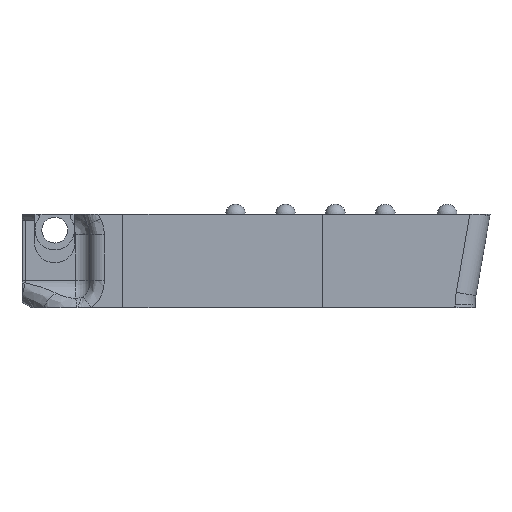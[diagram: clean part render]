
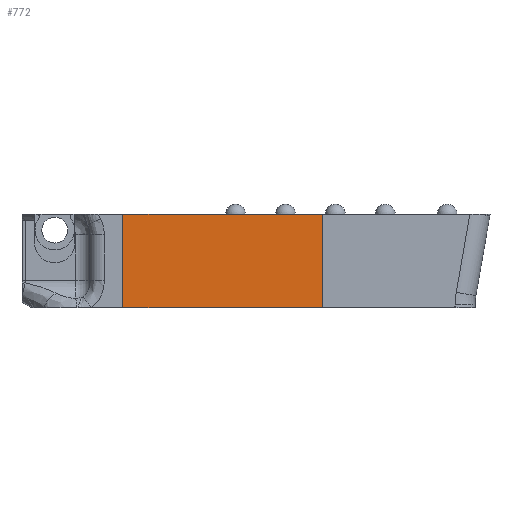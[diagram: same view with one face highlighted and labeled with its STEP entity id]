
A CAD part, front view. The second image highlights one B-rep face of the part: STEP entity #772.
In plain terms, the highlighted planar face has unit normal (0, -1, 0).
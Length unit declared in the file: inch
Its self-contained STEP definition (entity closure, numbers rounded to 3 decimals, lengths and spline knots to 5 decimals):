
#132 = CARTESIAN_POINT ( 'NONE',  ( 4.03265, -1.85855, -0.21577 ) ) ;
#195 = EDGE_CURVE ( 'NONE', #2408, #2262, #1029, .T. ) ;
#203 = EDGE_CURVE ( 'NONE', #3569, #3146, #998, .T. ) ;
#211 = DIRECTION ( 'NONE',  ( 1., 0., 0. ) ) ;
#310 = ORIENTED_EDGE ( 'NONE', *, *, #203, .T. ) ;
#409 = CARTESIAN_POINT ( 'NONE',  ( 4.03265, -1.85855, -0.21577 ) ) ;
#589 = FACE_OUTER_BOUND ( 'NONE', #4077, .T. ) ;
#772 = ADVANCED_FACE ( 'NONE', ( #589 ), #2715, .T. ) ;
#847 = AXIS2_PLACEMENT_3D ( 'NONE', #2646, #2638, #2623 ) ;
#848 = DIRECTION ( 'NONE',  ( 0., 0., 1. ) ) ;
#990 = VECTOR ( 'NONE', #4670, 39.37008 ) ;
#998 = LINE ( 'NONE', #3931, #990 ) ;
#1011 = VECTOR ( 'NONE', #848, 39.37008 ) ;
#1029 = LINE ( 'NONE', #4497, #1011 ) ;
#1628 = CARTESIAN_POINT ( 'NONE',  ( 5.60745, -1.85855, 0.5209 ) ) ;
#2085 = CARTESIAN_POINT ( 'NONE',  ( 5.60745, -1.85855, 0.5209 ) ) ;
#2233 = VECTOR ( 'NONE', #211, 39.37008 ) ;
#2247 = LINE ( 'NONE', #132, #2233 ) ;
#2262 = VERTEX_POINT ( 'NONE', #1628 ) ;
#2408 = VERTEX_POINT ( 'NONE', #2458 ) ;
#2458 = CARTESIAN_POINT ( 'NONE',  ( 5.60745, -1.85855, -0.21577 ) ) ;
#2623 = DIRECTION ( 'NONE',  ( 0., 0., -1. ) ) ;
#2638 = DIRECTION ( 'NONE',  ( 0., -1., 0. ) ) ;
#2646 = CARTESIAN_POINT ( 'NONE',  ( 0., -1.85855, 0. ) ) ;
#2715 = PLANE ( 'NONE',  #847 ) ;
#2955 = VECTOR ( 'NONE', #3206, 39.37008 ) ;
#3004 = LINE ( 'NONE', #2085, #2955 ) ;
#3146 = VERTEX_POINT ( 'NONE', #409 ) ;
#3206 = DIRECTION ( 'NONE',  ( -1., 0., 0. ) ) ;
#3261 = EDGE_CURVE ( 'NONE', #2262, #3569, #3004, .T. ) ;
#3402 = CARTESIAN_POINT ( 'NONE',  ( 4.03265, -1.85855, 0.5209 ) ) ;
#3569 = VERTEX_POINT ( 'NONE', #3402 ) ;
#3795 = EDGE_CURVE ( 'NONE', #3146, #2408, #2247, .T. ) ;
#3931 = CARTESIAN_POINT ( 'NONE',  ( 4.03265, -1.85855, 0.5209 ) ) ;
#4077 = EDGE_LOOP ( 'NONE', ( #4117, #310, #4263, #4296 ) ) ;
#4117 = ORIENTED_EDGE ( 'NONE', *, *, #3261, .T. ) ;
#4263 = ORIENTED_EDGE ( 'NONE', *, *, #3795, .T. ) ;
#4296 = ORIENTED_EDGE ( 'NONE', *, *, #195, .T. ) ;
#4497 = CARTESIAN_POINT ( 'NONE',  ( 5.60745, -1.85855, -0.21577 ) ) ;
#4670 = DIRECTION ( 'NONE',  ( 0., 0., -1. ) ) ;
